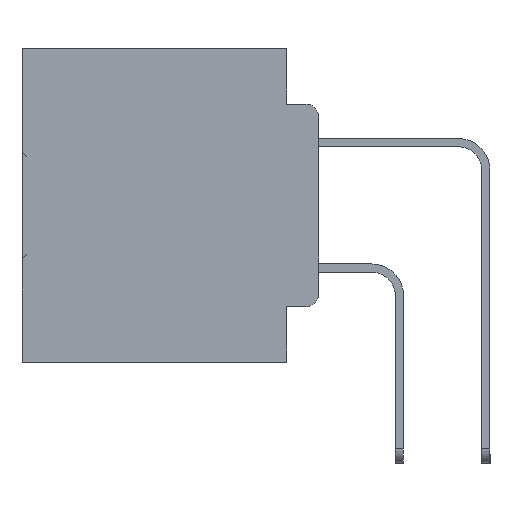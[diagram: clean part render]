
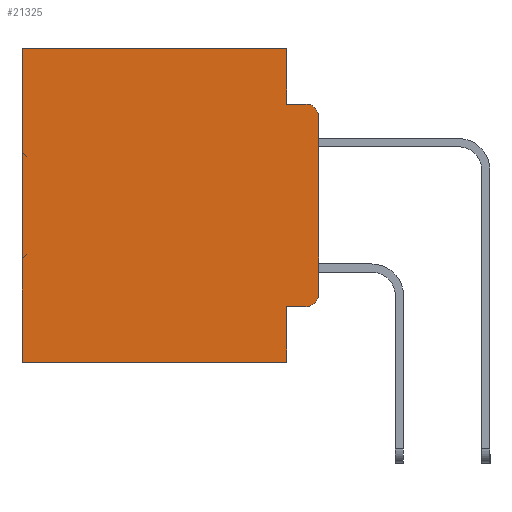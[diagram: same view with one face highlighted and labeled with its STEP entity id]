
A CAD part, left-side view. The second image highlights one B-rep face of the part: STEP entity #21325.
In plain terms, the highlighted planar face has unit normal (-1, 0, 0).
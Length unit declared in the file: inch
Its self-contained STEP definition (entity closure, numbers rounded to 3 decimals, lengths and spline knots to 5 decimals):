
#367 = CIRCLE ( 'NONE', #10732, 0.02 ) ;
#1603 = CARTESIAN_POINT ( 'NONE',  ( 0.298, 0.02, -0.1085 ) ) ;
#2042 = ORIENTED_EDGE ( 'NONE', *, *, #29502, .F. ) ;
#2125 = EDGE_CURVE ( 'NONE', #35946, #37165, #22282, .T. ) ;
#2369 = VECTOR ( 'NONE', #22165, 39.37008 ) ;
#2371 = VERTEX_POINT ( 'NONE', #24230 ) ;
#3161 = CARTESIAN_POINT ( 'NONE',  ( 0.298, 0., 0. ) ) ;
#4101 = EDGE_CURVE ( 'NONE', #37165, #37222, #32846, .T. ) ;
#4577 = DIRECTION ( 'NONE',  ( 0., 0., -1. ) ) ;
#6036 = EDGE_CURVE ( 'NONE', #7709, #32742, #10708, .T. ) ;
#6242 = ORIENTED_EDGE ( 'NONE', *, *, #19673, .T. ) ;
#6412 = ORIENTED_EDGE ( 'NONE', *, *, #29725, .T. ) ;
#7709 = VERTEX_POINT ( 'NONE', #22785 ) ;
#7770 = CARTESIAN_POINT ( 'NONE',  ( 0.298, 0.051, -0.4115 ) ) ;
#7828 = VECTOR ( 'NONE', #16205, 39.37008 ) ;
#8017 = ORIENTED_EDGE ( 'NONE', *, *, #2125, .F. ) ;
#8387 = CARTESIAN_POINT ( 'NONE',  ( 0.298, 0., -0.3915 ) ) ;
#9375 = CARTESIAN_POINT ( 'NONE',  ( 0.298, 0.02, -0.4115 ) ) ;
#9907 = VECTOR ( 'NONE', #20196, 39.37008 ) ;
#10708 = LINE ( 'NONE', #22399, #19331 ) ;
#10712 = VECTOR ( 'NONE', #18179, 39.37008 ) ;
#10732 = AXIS2_PLACEMENT_3D ( 'NONE', #30251, #12983, #33079 ) ;
#10899 = DIRECTION ( 'NONE',  ( 0., 0., -1. ) ) ;
#11205 = CARTESIAN_POINT ( 'NONE',  ( 0.298, 0.051, -0.0885 ) ) ;
#12238 = CARTESIAN_POINT ( 'NONE',  ( 0.298, 0.051, 0. ) ) ;
#12511 = ORIENTED_EDGE ( 'NONE', *, *, #6036, .F. ) ;
#12983 = DIRECTION ( 'NONE',  ( -1., 0., 0. ) ) ;
#13423 = ORIENTED_EDGE ( 'NONE', *, *, #15765, .T. ) ;
#13696 = CARTESIAN_POINT ( 'NONE',  ( 0.298, 0., 0. ) ) ;
#14196 = ORIENTED_EDGE ( 'NONE', *, *, #29992, .T. ) ;
#15765 = EDGE_CURVE ( 'NONE', #37033, #17314, #30003, .T. ) ;
#16205 = DIRECTION ( 'NONE',  ( 0., 0., -1. ) ) ;
#17127 = DIRECTION ( 'NONE',  ( 0., 0., -1. ) ) ;
#17314 = VERTEX_POINT ( 'NONE', #30897 ) ;
#17476 = CIRCLE ( 'NONE', #31263, 0.02 ) ;
#17705 = EDGE_CURVE ( 'NONE', #28295, #23186, #367, .T. ) ;
#18179 = DIRECTION ( 'NONE',  ( 0., 1., 0. ) ) ;
#18851 = VECTOR ( 'NONE', #20566, 39.37008 ) ;
#19331 = VECTOR ( 'NONE', #31688, 39.37008 ) ;
#19532 = PLANE ( 'NONE',  #29898 ) ;
#19673 = EDGE_CURVE ( 'NONE', #7709, #28295, #25496, .T. ) ;
#19785 = LINE ( 'NONE', #3161, #18851 ) ;
#19866 = ORIENTED_EDGE ( 'NONE', *, *, #17705, .T. ) ;
#19930 = CARTESIAN_POINT ( 'NONE',  ( 0.298, 0., 0. ) ) ;
#20196 = DIRECTION ( 'NONE',  ( 0., -1., 0. ) ) ;
#20287 = CARTESIAN_POINT ( 'NONE',  ( 0.298, 0.051, 0. ) ) ;
#20566 = DIRECTION ( 'NONE',  ( 0., 1., 0. ) ) ;
#20957 = CARTESIAN_POINT ( 'NONE',  ( 0.298, 0., -0.5 ) ) ;
#21088 = DIRECTION ( 'NONE',  ( 0., 0., -1. ) ) ;
#21325 = ADVANCED_FACE ( 'NONE', ( #21812 ), #19532, .F. ) ;
#21456 = VECTOR ( 'NONE', #21088, 39.37008 ) ;
#21812 = FACE_OUTER_BOUND ( 'NONE', #30649, .T. ) ;
#21920 = DIRECTION ( 'NONE',  ( -1., 0., 0. ) ) ;
#22157 = VECTOR ( 'NONE', #17127, 39.37008 ) ;
#22165 = DIRECTION ( 'NONE',  ( 0., -1., 0. ) ) ;
#22282 = LINE ( 'NONE', #20287, #7828 ) ;
#22399 = CARTESIAN_POINT ( 'NONE',  ( 0.298, 0.051, 0. ) ) ;
#22785 = CARTESIAN_POINT ( 'NONE',  ( 0.298, 0.051, -0.4115 ) ) ;
#23186 = VERTEX_POINT ( 'NONE', #8387 ) ;
#23739 = CARTESIAN_POINT ( 'NONE',  ( 0.298, 0.02, -0.0885 ) ) ;
#24230 = CARTESIAN_POINT ( 'NONE',  ( 0.298, 0., -0.1085 ) ) ;
#25496 = LINE ( 'NONE', #7770, #2369 ) ;
#25862 = CARTESIAN_POINT ( 'NONE',  ( 0.298, 0.051, -0.0885 ) ) ;
#26060 = LINE ( 'NONE', #20957, #10712 ) ;
#28025 = CARTESIAN_POINT ( 'NONE',  ( 0.298, 0.473, 0. ) ) ;
#28081 = EDGE_CURVE ( 'NONE', #2371, #23186, #29788, .T. ) ;
#28181 = DIRECTION ( 'NONE',  ( 1., 0., 0. ) ) ;
#28295 = VERTEX_POINT ( 'NONE', #9375 ) ;
#29502 = EDGE_CURVE ( 'NONE', #32742, #17314, #26060, .T. ) ;
#29725 = EDGE_CURVE ( 'NONE', #35946, #37033, #19785, .T. ) ;
#29788 = LINE ( 'NONE', #19930, #22157 ) ;
#29898 = AXIS2_PLACEMENT_3D ( 'NONE', #13696, #28181, #10899 ) ;
#29992 = EDGE_CURVE ( 'NONE', #2371, #37222, #17476, .T. ) ;
#30003 = LINE ( 'NONE', #32471, #21456 ) ;
#30251 = CARTESIAN_POINT ( 'NONE',  ( 0.298, 0.02, -0.3915 ) ) ;
#30398 = ORIENTED_EDGE ( 'NONE', *, *, #28081, .F. ) ;
#30649 = EDGE_LOOP ( 'NONE', ( #30398, #14196, #36985, #8017, #6412, #13423, #2042, #12511, #6242, #19866 ) ) ;
#30897 = CARTESIAN_POINT ( 'NONE',  ( 0.298, 0.473, -0.5 ) ) ;
#31263 = AXIS2_PLACEMENT_3D ( 'NONE', #1603, #21920, #4577 ) ;
#31688 = DIRECTION ( 'NONE',  ( 0., 0., -1. ) ) ;
#32471 = CARTESIAN_POINT ( 'NONE',  ( 0.298, 0.473, 0. ) ) ;
#32742 = VERTEX_POINT ( 'NONE', #35527 ) ;
#32846 = LINE ( 'NONE', #11205, #9907 ) ;
#33079 = DIRECTION ( 'NONE',  ( 0., 0., -1. ) ) ;
#35527 = CARTESIAN_POINT ( 'NONE',  ( 0.298, 0.051, -0.5 ) ) ;
#35946 = VERTEX_POINT ( 'NONE', #12238 ) ;
#36985 = ORIENTED_EDGE ( 'NONE', *, *, #4101, .F. ) ;
#37033 = VERTEX_POINT ( 'NONE', #28025 ) ;
#37165 = VERTEX_POINT ( 'NONE', #25862 ) ;
#37222 = VERTEX_POINT ( 'NONE', #23739 ) ;
